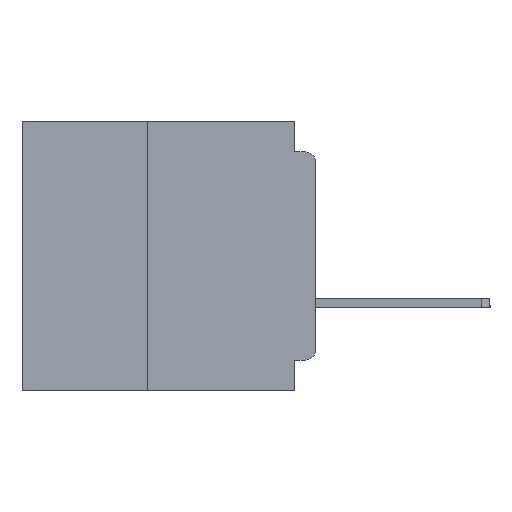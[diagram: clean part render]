
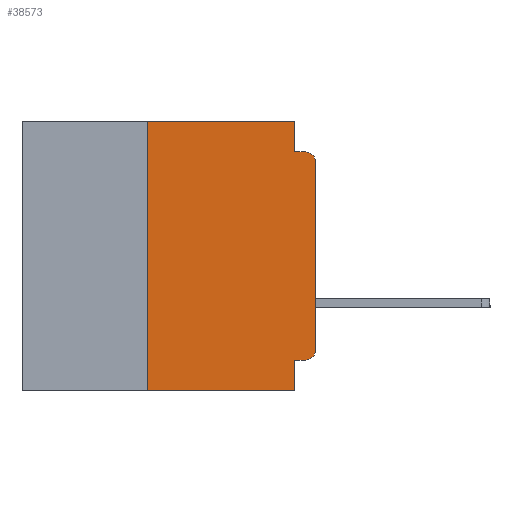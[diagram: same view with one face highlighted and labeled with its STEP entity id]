
A CAD part, left-side view. The second image highlights one B-rep face of the part: STEP entity #38573.
In plain terms, the highlighted planar face has unit normal (-1, 0, 0).
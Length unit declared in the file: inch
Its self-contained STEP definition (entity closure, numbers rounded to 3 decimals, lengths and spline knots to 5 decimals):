
#389 = AXIS2_PLACEMENT_3D ( 'NONE', #44989, #15219, #49941 ) ;
#3648 = LINE ( 'NONE', #63257, #28443 ) ;
#3834 = CARTESIAN_POINT ( 'NONE',  ( 0., 0.031, 0. ) ) ;
#5188 = FACE_OUTER_BOUND ( 'NONE', #51103, .T. ) ;
#5608 = CARTESIAN_POINT ( 'NONE',  ( 0., 0.031, -0.4 ) ) ;
#5634 = EDGE_CURVE ( 'NONE', #31764, #18489, #57733, .T. ) ;
#6150 = VERTEX_POINT ( 'NONE', #37795 ) ;
#6960 = AXIS2_PLACEMENT_3D ( 'NONE', #39642, #9908, #44618 ) ;
#6990 = CARTESIAN_POINT ( 'NONE',  ( 0., 0.015, -0.045 ) ) ;
#8483 = LINE ( 'NONE', #22027, #10052 ) ;
#9085 = DIRECTION ( 'NONE',  ( 0., 0., 1. ) ) ;
#9885 = VECTOR ( 'NONE', #35329, 39.37008 ) ;
#9908 = DIRECTION ( 'NONE',  ( -1., 0., 0. ) ) ;
#10052 = VECTOR ( 'NONE', #51726, 39.37008 ) ;
#11324 = EDGE_CURVE ( 'NONE', #33604, #61496, #31827, .T. ) ;
#11387 = ORIENTED_EDGE ( 'NONE', *, *, #11324, .F. ) ;
#11410 = LINE ( 'NONE', #5608, #9885 ) ;
#12047 = EDGE_CURVE ( 'NONE', #27898, #30251, #34155, .T. ) ;
#13115 = CARTESIAN_POINT ( 'NONE',  ( 0., 0.031, -0.045 ) ) ;
#13573 = ORIENTED_EDGE ( 'NONE', *, *, #50380, .F. ) ;
#13787 = EDGE_CURVE ( 'NONE', #6150, #14701, #48303, .T. ) ;
#13883 = VECTOR ( 'NONE', #9085, 39.37008 ) ;
#14701 = VERTEX_POINT ( 'NONE', #17457 ) ;
#14865 = VECTOR ( 'NONE', #42160, 39.37008 ) ;
#15219 = DIRECTION ( 'NONE',  ( -1., 0., 0. ) ) ;
#17138 = AXIS2_PLACEMENT_3D ( 'NONE', #43148, #28400, #63052 ) ;
#17457 = CARTESIAN_POINT ( 'NONE',  ( 0., 0.031, -0.355 ) ) ;
#18489 = VERTEX_POINT ( 'NONE', #13115 ) ;
#19302 = ORIENTED_EDGE ( 'NONE', *, *, #44730, .F. ) ;
#19929 = CIRCLE ( 'NONE', #6960, 0.015 ) ;
#19987 = DIRECTION ( 'NONE',  ( 0., 1., 0. ) ) ;
#20921 = CARTESIAN_POINT ( 'NONE',  ( 0., 0.031, -0.4 ) ) ;
#22027 = CARTESIAN_POINT ( 'NONE',  ( 0., 0., -0.045 ) ) ;
#23221 = ORIENTED_EDGE ( 'NONE', *, *, #13787, .F. ) ;
#23623 = DIRECTION ( 'NONE',  ( 0., -1., 0. ) ) ;
#25005 = ORIENTED_EDGE ( 'NONE', *, *, #35837, .T. ) ;
#27898 = VERTEX_POINT ( 'NONE', #35254 ) ;
#28400 = DIRECTION ( 'NONE',  ( 1., 0., 0. ) ) ;
#28443 = VECTOR ( 'NONE', #23623, 39.37008 ) ;
#29057 = CARTESIAN_POINT ( 'NONE',  ( 0., 0.25, -0.4 ) ) ;
#29568 = ORIENTED_EDGE ( 'NONE', *, *, #38583, .T. ) ;
#29880 = ORIENTED_EDGE ( 'NONE', *, *, #5634, .F. ) ;
#30251 = VERTEX_POINT ( 'NONE', #6990 ) ;
#31025 = VERTEX_POINT ( 'NONE', #20921 ) ;
#31764 = VERTEX_POINT ( 'NONE', #56366 ) ;
#31827 = LINE ( 'NONE', #29057, #13883 ) ;
#32963 = VECTOR ( 'NONE', #58187, 39.37008 ) ;
#33604 = VERTEX_POINT ( 'NONE', #39661 ) ;
#34155 = CIRCLE ( 'NONE', #389, 0.015 ) ;
#35254 = CARTESIAN_POINT ( 'NONE',  ( 0., 0., -0.06 ) ) ;
#35329 = DIRECTION ( 'NONE',  ( 0., 0., -1. ) ) ;
#35837 = EDGE_CURVE ( 'NONE', #36467, #27898, #47420, .T. ) ;
#36467 = VERTEX_POINT ( 'NONE', #37546 ) ;
#37546 = CARTESIAN_POINT ( 'NONE',  ( 0., 0., -0.34 ) ) ;
#37795 = CARTESIAN_POINT ( 'NONE',  ( 0., 0.015, -0.355 ) ) ;
#38284 = CARTESIAN_POINT ( 'NONE',  ( 0., 0., 0. ) ) ;
#38573 = ADVANCED_FACE ( 'NONE', ( #5188 ), #48098, .F. ) ;
#38583 = EDGE_CURVE ( 'NONE', #33604, #31025, #3648, .T. ) ;
#39642 = CARTESIAN_POINT ( 'NONE',  ( 0., 0.015, -0.34 ) ) ;
#39661 = CARTESIAN_POINT ( 'NONE',  ( 0., 0.25, -0.4 ) ) ;
#41311 = LINE ( 'NONE', #47130, #14865 ) ;
#42160 = DIRECTION ( 'NONE',  ( 0., -1., 0. ) ) ;
#43148 = CARTESIAN_POINT ( 'NONE',  ( 0., 0.437, 0. ) ) ;
#44618 = DIRECTION ( 'NONE',  ( 0., 0., -1. ) ) ;
#44730 = EDGE_CURVE ( 'NONE', #14701, #31025, #11410, .T. ) ;
#44989 = CARTESIAN_POINT ( 'NONE',  ( 0., 0.015, -0.06 ) ) ;
#46768 = VECTOR ( 'NONE', #19987, 39.37008 ) ;
#46958 = ORIENTED_EDGE ( 'NONE', *, *, #12047, .T. ) ;
#47130 = CARTESIAN_POINT ( 'NONE',  ( 0., 0.437, 0. ) ) ;
#47420 = LINE ( 'NONE', #38284, #60591 ) ;
#48098 = PLANE ( 'NONE',  #17138 ) ;
#48303 = LINE ( 'NONE', #54673, #46768 ) ;
#49941 = DIRECTION ( 'NONE',  ( 0., 0., -1. ) ) ;
#50380 = EDGE_CURVE ( 'NONE', #18489, #30251, #8483, .T. ) ;
#51103 = EDGE_LOOP ( 'NONE', ( #25005, #46958, #13573, #29880, #59073, #11387, #29568, #19302, #23221, #51189 ) ) ;
#51189 = ORIENTED_EDGE ( 'NONE', *, *, #55551, .T. ) ;
#51726 = DIRECTION ( 'NONE',  ( 0., -1., 0. ) ) ;
#54673 = CARTESIAN_POINT ( 'NONE',  ( 0., 0., -0.355 ) ) ;
#55551 = EDGE_CURVE ( 'NONE', #6150, #36467, #19929, .T. ) ;
#56366 = CARTESIAN_POINT ( 'NONE',  ( 0., 0.031, 0. ) ) ;
#56542 = CARTESIAN_POINT ( 'NONE',  ( 0., 0.25, 0. ) ) ;
#57733 = LINE ( 'NONE', #3834, #32963 ) ;
#58187 = DIRECTION ( 'NONE',  ( 0., 0., -1. ) ) ;
#58862 = EDGE_CURVE ( 'NONE', #61496, #31764, #41311, .T. ) ;
#59073 = ORIENTED_EDGE ( 'NONE', *, *, #58862, .F. ) ;
#60591 = VECTOR ( 'NONE', #62934, 39.37008 ) ;
#61496 = VERTEX_POINT ( 'NONE', #56542 ) ;
#62934 = DIRECTION ( 'NONE',  ( 0., 0., 1. ) ) ;
#63052 = DIRECTION ( 'NONE',  ( 0., 0., -1. ) ) ;
#63257 = CARTESIAN_POINT ( 'NONE',  ( 0., 0.437, -0.4 ) ) ;
